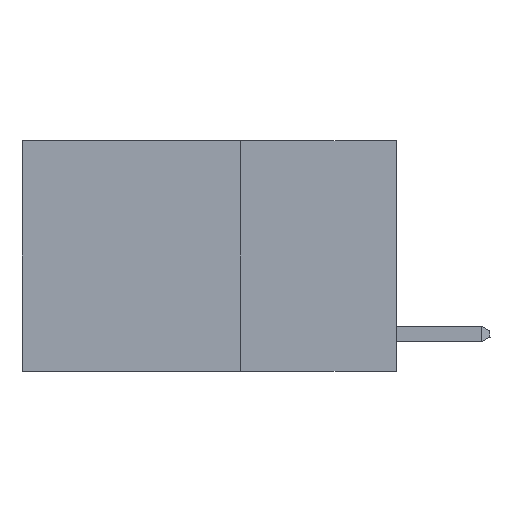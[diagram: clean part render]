
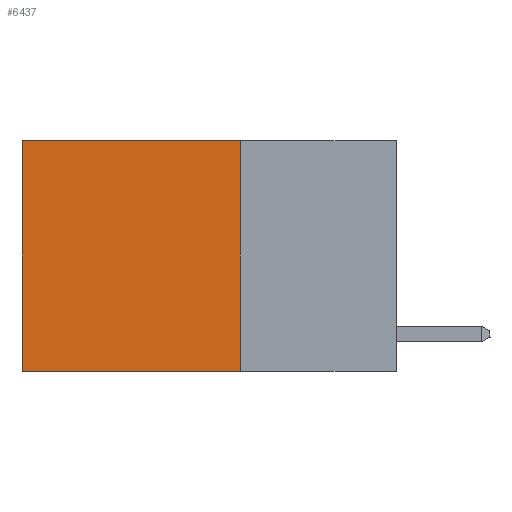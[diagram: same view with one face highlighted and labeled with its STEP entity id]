
A CAD part, left-side view. The second image highlights one B-rep face of the part: STEP entity #6437.
In plain terms, the highlighted planar face has unit normal (-1, 0, 0).
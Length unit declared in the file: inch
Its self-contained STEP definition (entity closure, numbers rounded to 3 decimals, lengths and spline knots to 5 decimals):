
#431 = VECTOR ( 'NONE', #8798, 39.37008 ) ;
#1216 = CARTESIAN_POINT ( 'NONE',  ( 0.2625, 0.6, 0. ) ) ;
#1417 = LINE ( 'NONE', #1216, #12009 ) ;
#1484 = AXIS2_PLACEMENT_3D ( 'NONE', #1992, #10095, #1794 ) ;
#1673 = ORIENTED_EDGE ( 'NONE', *, *, #5697, .T. ) ;
#1690 = CARTESIAN_POINT ( 'NONE',  ( 0.2625, 0.6, -0.37 ) ) ;
#1794 = DIRECTION ( 'NONE',  ( 0., 0., -1. ) ) ;
#1895 = CARTESIAN_POINT ( 'NONE',  ( 0.2625, 0.25, 0. ) ) ;
#1992 = CARTESIAN_POINT ( 'NONE',  ( 0.2625, 0.25, 0. ) ) ;
#2205 = EDGE_CURVE ( 'NONE', #11112, #9752, #5335, .T. ) ;
#2736 = VERTEX_POINT ( 'NONE', #1690 ) ;
#3125 = LINE ( 'NONE', #1895, #9706 ) ;
#3224 = VERTEX_POINT ( 'NONE', #9592 ) ;
#3824 = EDGE_CURVE ( 'NONE', #11112, #3224, #3125, .T. ) ;
#5335 = LINE ( 'NONE', #8422, #8236 ) ;
#5697 = EDGE_CURVE ( 'NONE', #3224, #2736, #1417, .T. ) ;
#6023 = CARTESIAN_POINT ( 'NONE',  ( 0.2625, 0.25, -0.37 ) ) ;
#6437 = ADVANCED_FACE ( 'NONE', ( #7126 ), #13156, .F. ) ;
#6651 = CARTESIAN_POINT ( 'NONE',  ( 0.2625, 0.25, 0. ) ) ;
#7024 = LINE ( 'NONE', #6023, #431 ) ;
#7126 = FACE_OUTER_BOUND ( 'NONE', #10475, .T. ) ;
#7577 = DIRECTION ( 'NONE',  ( 0., 0., -1. ) ) ;
#7644 = ORIENTED_EDGE ( 'NONE', *, *, #3824, .T. ) ;
#8123 = EDGE_CURVE ( 'NONE', #9752, #2736, #7024, .T. ) ;
#8143 = DIRECTION ( 'NONE',  ( 0., 0., -1. ) ) ;
#8236 = VECTOR ( 'NONE', #8143, 39.37008 ) ;
#8422 = CARTESIAN_POINT ( 'NONE',  ( 0.2625, 0.25, 0. ) ) ;
#8744 = CARTESIAN_POINT ( 'NONE',  ( 0.2625, 0.25, -0.37 ) ) ;
#8798 = DIRECTION ( 'NONE',  ( 0., 1., 0. ) ) ;
#9566 = ORIENTED_EDGE ( 'NONE', *, *, #2205, .F. ) ;
#9592 = CARTESIAN_POINT ( 'NONE',  ( 0.2625, 0.6, 0. ) ) ;
#9706 = VECTOR ( 'NONE', #13280, 39.37008 ) ;
#9752 = VERTEX_POINT ( 'NONE', #8744 ) ;
#10095 = DIRECTION ( 'NONE',  ( 1., 0., 0. ) ) ;
#10475 = EDGE_LOOP ( 'NONE', ( #1673, #11479, #9566, #7644 ) ) ;
#11112 = VERTEX_POINT ( 'NONE', #6651 ) ;
#11479 = ORIENTED_EDGE ( 'NONE', *, *, #8123, .F. ) ;
#12009 = VECTOR ( 'NONE', #7577, 39.37008 ) ;
#13156 = PLANE ( 'NONE',  #1484 ) ;
#13280 = DIRECTION ( 'NONE',  ( 0., 1., 0. ) ) ;
